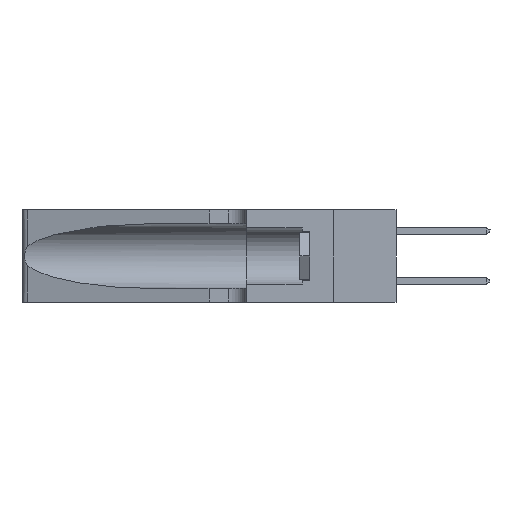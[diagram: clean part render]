
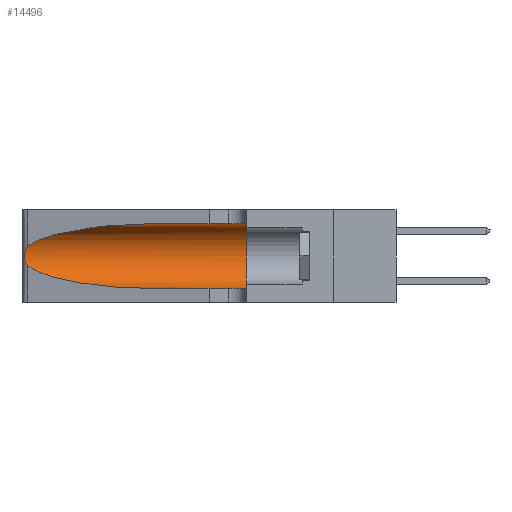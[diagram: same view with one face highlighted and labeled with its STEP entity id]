
A CAD part, left-side view. The second image highlights one B-rep face of the part: STEP entity #14496.
In plain terms, the highlighted cylindrical face has radius 3.308 mm (diameter 6.617 mm), a partial arc.
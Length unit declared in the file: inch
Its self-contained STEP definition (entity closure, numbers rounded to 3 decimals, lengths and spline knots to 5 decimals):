
#503 = CARTESIAN_POINT ( 'NONE',  ( 0.26075, 1.23896, 0.178 ) ) ;
#1508 = ORIENTED_EDGE ( 'NONE', *, *, #16046, .T. ) ;
#1861 = ORIENTED_EDGE ( 'NONE', *, *, #11359, .F. ) ;
#1997 = CARTESIAN_POINT ( 'NONE',  ( 0.25856, 1.23593, 0.16098 ) ) ;
#2269 = CARTESIAN_POINT ( 'NONE',  ( 0.1305, 1.61858, 0.31525 ) ) ;
#2542 =( BOUNDED_CURVE ( )  B_SPLINE_CURVE ( 3, ( #38702, #38253, #8054, #42096 ),
 .UNSPECIFIED., .F., .T. ) 
 B_SPLINE_CURVE_WITH_KNOTS ( ( 4, 4 ),
 ( 3.44316, 4.71239 ),
 .UNSPECIFIED. ) 
 CURVE ( )  GEOMETRIC_REPRESENTATION_ITEM ( )  RATIONAL_B_SPLINE_CURVE ( ( 1., 0.87, 0.87, 1. ) ) 
 REPRESENTATION_ITEM ( '' )  );
#3256 = CARTESIAN_POINT ( 'NONE',  ( 0.1305, 0.35, 0.185 ) ) ;
#3311 =( BOUNDED_CURVE ( )  B_SPLINE_CURVE ( 3, ( #36672, #9893, #16633, #6668 ),
 .UNSPECIFIED., .F., .F. ) 
 B_SPLINE_CURVE_WITH_KNOTS ( ( 4, 4 ),
 ( 1.5708, 2.84003 ),
 .UNSPECIFIED. ) 
 CURVE ( )  GEOMETRIC_REPRESENTATION_ITEM ( )  RATIONAL_B_SPLINE_CURVE ( ( 1., 0.87, 0.87, 1. ) ) 
 REPRESENTATION_ITEM ( '' )  );
#3845 = CARTESIAN_POINT ( 'NONE',  ( 0.1305, 0.72297, 0.31525 ) ) ;
#4166 = CARTESIAN_POINT ( 'NONE',  ( 0.1305, 0.72297, 0.05475 ) ) ;
#4362 = CARTESIAN_POINT ( 'NONE',  ( 0.25487, 1.22718, 0.14631 ) ) ;
#4801 = CARTESIAN_POINT ( 'NONE',  ( 0.25487, 1.22718, 0.14631 ) ) ;
#5931 = CARTESIAN_POINT ( 'NONE',  ( 0.26017, 1.23833, 0.17102 ) ) ;
#6611 = CARTESIAN_POINT ( 'NONE',  ( 0.1305, 0.35, 0.05475 ) ) ;
#6668 = CARTESIAN_POINT ( 'NONE',  ( 0.25487, 1.22718, 0.22369 ) ) ;
#8054 = CARTESIAN_POINT ( 'NONE',  ( 0.18966, 0.96281, 0.05475 ) ) ;
#8107 = VECTOR ( 'NONE', #39886, 39.37008 ) ;
#9008 = CARTESIAN_POINT ( 'NONE',  ( 0.25789, 1.23486, 0.15765 ) ) ;
#9056 = CARTESIAN_POINT ( 'NONE',  ( 0.25854, 1.2359, 0.20912 ) ) ;
#9884 = DIRECTION ( 'NONE',  ( 0., -1., 0. ) ) ;
#9893 = CARTESIAN_POINT ( 'NONE',  ( 0.18966, 0.96281, 0.31525 ) ) ;
#10147 = VERTEX_POINT ( 'NONE', #22595 ) ;
#11229 = CYLINDRICAL_SURFACE ( 'NONE', #12687, 0.13025 ) ;
#11359 = EDGE_CURVE ( 'NONE', #10147, #32965, #40792, .T. ) ;
#12687 = AXIS2_PLACEMENT_3D ( 'NONE', #27084, #9884, #20033 ) ;
#13446 = VERTEX_POINT ( 'NONE', #4166 ) ;
#14426 = LINE ( 'NONE', #23234, #28116 ) ;
#14496 = ADVANCED_FACE ( 'NONE', ( #38636 ), #11229, .F. ) ;
#14511 = VERTEX_POINT ( 'NONE', #3845 ) ;
#14697 = DIRECTION ( 'NONE',  ( 0., 0., 1. ) ) ;
#16046 = EDGE_CURVE ( 'NONE', #19240, #38361, #41645, .T. ) ;
#16633 = CARTESIAN_POINT ( 'NONE',  ( 0.2373, 1.15595, 0.28018 ) ) ;
#18333 = CARTESIAN_POINT ( 'NONE',  ( 0.25639, 1.23186, 0.15144 ) ) ;
#18691 = ORIENTED_EDGE ( 'NONE', *, *, #31128, .T. ) ;
#18781 = CARTESIAN_POINT ( 'NONE',  ( 0.25787, 1.23484, 0.2124 ) ) ;
#19240 = VERTEX_POINT ( 'NONE', #37652 ) ;
#19406 = CARTESIAN_POINT ( 'NONE',  ( 0.25555, 1.22993, 0.14849 ) ) ;
#19776 = CARTESIAN_POINT ( 'NONE',  ( 0.26075, 1.23896, 0.19203 ) ) ;
#20033 = DIRECTION ( 'NONE',  ( 0., 0., -1. ) ) ;
#20501 = ORIENTED_EDGE ( 'NONE', *, *, #24694, .T. ) ;
#22595 = CARTESIAN_POINT ( 'NONE',  ( 0.1305, 0.35, 0.31525 ) ) ;
#23234 = CARTESIAN_POINT ( 'NONE',  ( 0.1305, 1.61858, 0.05475 ) ) ;
#24694 = EDGE_CURVE ( 'NONE', #14511, #19240, #3311, .T. ) ;
#27084 = CARTESIAN_POINT ( 'NONE',  ( 0.1305, 1.61858, 0.185 ) ) ;
#28116 = VECTOR ( 'NONE', #33355, 39.37008 ) ;
#30065 = AXIS2_PLACEMENT_3D ( 'NONE', #3256, #42676, #14697 ) ;
#31128 = EDGE_CURVE ( 'NONE', #38361, #13446, #2542, .T. ) ;
#32461 = CARTESIAN_POINT ( 'NONE',  ( 0.25487, 1.22718, 0.22369 ) ) ;
#32932 = EDGE_CURVE ( 'NONE', #13446, #32965, #14426, .T. ) ;
#32965 = VERTEX_POINT ( 'NONE', #6611 ) ;
#33355 = DIRECTION ( 'NONE',  ( 0., -1., 0. ) ) ;
#34970 = LINE ( 'NONE', #2269, #8107 ) ;
#35681 = ORIENTED_EDGE ( 'NONE', *, *, #32932, .T. ) ;
#36672 = CARTESIAN_POINT ( 'NONE',  ( 0.1305, 0.72297, 0.31525 ) ) ;
#37263 = EDGE_CURVE ( 'NONE', #14511, #10147, #34970, .T. ) ;
#37652 = CARTESIAN_POINT ( 'NONE',  ( 0.25487, 1.22718, 0.22369 ) ) ;
#37869 = EDGE_LOOP ( 'NONE', ( #20501, #1508, #18691, #35681, #1861, #38606 ) ) ;
#38253 = CARTESIAN_POINT ( 'NONE',  ( 0.2373, 1.15595, 0.08982 ) ) ;
#38361 = VERTEX_POINT ( 'NONE', #4801 ) ;
#38606 = ORIENTED_EDGE ( 'NONE', *, *, #37263, .F. ) ;
#38636 = FACE_OUTER_BOUND ( 'NONE', #37869, .T. ) ;
#38702 = CARTESIAN_POINT ( 'NONE',  ( 0.25487, 1.22718, 0.14631 ) ) ;
#39108 = CARTESIAN_POINT ( 'NONE',  ( 0.25639, 1.23184, 0.21858 ) ) ;
#39886 = DIRECTION ( 'NONE',  ( 0., -1., 0. ) ) ;
#40792 = CIRCLE ( 'NONE', #30065, 0.13025 ) ;
#41645 = B_SPLINE_CURVE_WITH_KNOTS ( 'NONE', 3,
 ( #32461, #42941, #39108, #18781, #9056, #42497, #19776, #503, #5931, #1997, #9008, #18333, #19406, #4362 ),
 .UNSPECIFIED., .F., .F.,
 ( 4, 2, 2, 2, 2, 2, 4 ),
 ( 0., 0.00027, 0.00053, 0.00107, 0.0016, 0.00187, 0.00214 ),
 .UNSPECIFIED. ) ;
#42096 = CARTESIAN_POINT ( 'NONE',  ( 0.1305, 0.72297, 0.05475 ) ) ;
#42497 = CARTESIAN_POINT ( 'NONE',  ( 0.26018, 1.23835, 0.19895 ) ) ;
#42676 = DIRECTION ( 'NONE',  ( 0., 1., 0. ) ) ;
#42941 = CARTESIAN_POINT ( 'NONE',  ( 0.25555, 1.22994, 0.2215 ) ) ;
